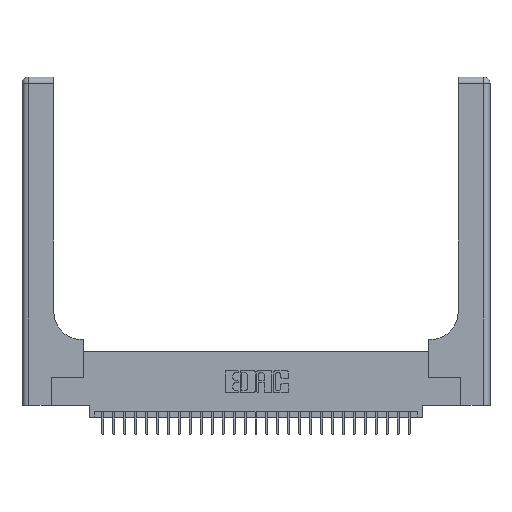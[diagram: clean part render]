
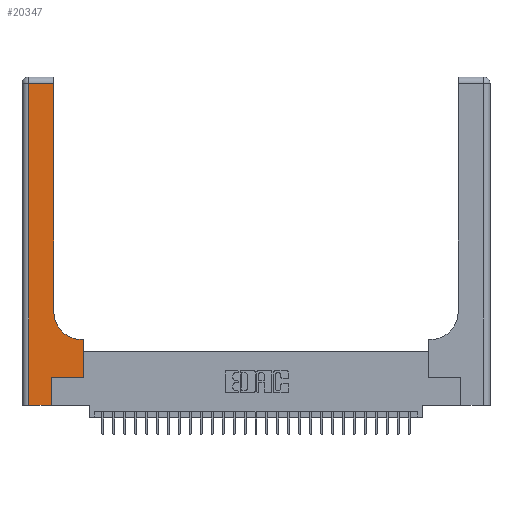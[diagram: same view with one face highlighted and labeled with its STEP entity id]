
A CAD part, top view. The second image highlights one B-rep face of the part: STEP entity #20347.
In plain terms, the highlighted planar face has unit normal (0, 0, 1).
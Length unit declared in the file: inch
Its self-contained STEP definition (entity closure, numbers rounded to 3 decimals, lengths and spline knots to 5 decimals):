
#326 = LINE ( 'NONE', #29440, #7261 ) ;
#518 = EDGE_CURVE ( 'NONE', #10290, #24856, #24675, .T. ) ;
#959 = LINE ( 'NONE', #28131, #12594 ) ;
#1615 = VECTOR ( 'NONE', #16192, 39.37008 ) ;
#1646 = VECTOR ( 'NONE', #24032, 39.37008 ) ;
#2129 = LINE ( 'NONE', #29507, #24504 ) ;
#3567 = PLANE ( 'NONE',  #21079 ) ;
#3671 = DIRECTION ( 'NONE',  ( 0., 0., -1. ) ) ;
#4589 = DIRECTION ( 'NONE',  ( 0., 1., 0. ) ) ;
#5098 = VERTEX_POINT ( 'NONE', #20747 ) ;
#5239 = AXIS2_PLACEMENT_3D ( 'NONE', #12744, #28800, #15045 ) ;
#5440 = VERTEX_POINT ( 'NONE', #18250 ) ;
#5540 = VERTEX_POINT ( 'NONE', #24027 ) ;
#5612 = CARTESIAN_POINT ( 'NONE',  ( 0.5585, 0.25, 0.37 ) ) ;
#5818 = FACE_OUTER_BOUND ( 'NONE', #27061, .T. ) ;
#6309 = VECTOR ( 'NONE', #28393, 39.37008 ) ;
#6556 = DIRECTION ( 'NONE',  ( -1., 0., 0. ) ) ;
#6905 = CARTESIAN_POINT ( 'NONE',  ( 0.269, 0.25, 0.37 ) ) ;
#7261 = VECTOR ( 'NONE', #15687, 39.37008 ) ;
#7595 = LINE ( 'NONE', #15906, #19853 ) ;
#7803 = LINE ( 'NONE', #6905, #1615 ) ;
#7983 = ORIENTED_EDGE ( 'NONE', *, *, #24202, .T. ) ;
#8025 = ORIENTED_EDGE ( 'NONE', *, *, #20539, .T. ) ;
#8749 = VERTEX_POINT ( 'NONE', #12777 ) ;
#9115 = ORIENTED_EDGE ( 'NONE', *, *, #15377, .T. ) ;
#9127 = ORIENTED_EDGE ( 'NONE', *, *, #18694, .T. ) ;
#9358 = EDGE_CURVE ( 'NONE', #5440, #18376, #28609, .T. ) ;
#10228 = ORIENTED_EDGE ( 'NONE', *, *, #9358, .T. ) ;
#10290 = VERTEX_POINT ( 'NONE', #22815 ) ;
#12074 = DIRECTION ( 'NONE',  ( 0., 1., 0. ) ) ;
#12594 = VECTOR ( 'NONE', #12074, 39.37008 ) ;
#12744 = CARTESIAN_POINT ( 'NONE',  ( 0.5415, 0.85, 0.37 ) ) ;
#12777 = CARTESIAN_POINT ( 'NONE',  ( 0.2915, 2.94, 0.37 ) ) ;
#13339 = CARTESIAN_POINT ( 'NONE',  ( 0.269, 0., 0.37 ) ) ;
#13676 = EDGE_CURVE ( 'NONE', #23272, #5098, #24753, .T. ) ;
#13821 = ORIENTED_EDGE ( 'NONE', *, *, #518, .T. ) ;
#13868 = LINE ( 'NONE', #18434, #26075 ) ;
#14112 = EDGE_CURVE ( 'NONE', #5540, #23272, #7803, .T. ) ;
#14633 = CARTESIAN_POINT ( 'NONE',  ( 0.5585, 0.25, 0.37 ) ) ;
#14650 = CARTESIAN_POINT ( 'NONE',  ( 0., 0., 0.37 ) ) ;
#15045 = DIRECTION ( 'NONE',  ( 1., 0., 0. ) ) ;
#15209 = CARTESIAN_POINT ( 'NONE',  ( 0., 3., 0.37 ) ) ;
#15377 = EDGE_CURVE ( 'NONE', #18376, #8749, #959, .T. ) ;
#15687 = DIRECTION ( 'NONE',  ( 0., -1., 0. ) ) ;
#15906 = CARTESIAN_POINT ( 'NONE',  ( 0., 2.94, 0.37 ) ) ;
#16192 = DIRECTION ( 'NONE',  ( 1., 0., 0. ) ) ;
#18250 = CARTESIAN_POINT ( 'NONE',  ( 0.5415, 0.6, 0.37 ) ) ;
#18376 = VERTEX_POINT ( 'NONE', #26567 ) ;
#18434 = CARTESIAN_POINT ( 'NONE',  ( 0.269, 0., 0.37 ) ) ;
#18694 = EDGE_CURVE ( 'NONE', #24856, #5540, #13868, .T. ) ;
#19668 = CARTESIAN_POINT ( 'NONE',  ( 0.06, 2.94, 0.37 ) ) ;
#19828 = DIRECTION ( 'NONE',  ( -1., 0., 0. ) ) ;
#19853 = VECTOR ( 'NONE', #29660, 39.37008 ) ;
#20347 = ADVANCED_FACE ( 'NONE', ( #5818 ), #3567, .F. ) ;
#20539 = EDGE_CURVE ( 'NONE', #8749, #21551, #7595, .T. ) ;
#20747 = CARTESIAN_POINT ( 'NONE',  ( 0.5585, 0.6, 0.37 ) ) ;
#21079 = AXIS2_PLACEMENT_3D ( 'NONE', #15209, #3671, #19828 ) ;
#21551 = VERTEX_POINT ( 'NONE', #19668 ) ;
#22815 = CARTESIAN_POINT ( 'NONE',  ( 0.06, 0., 0.37 ) ) ;
#23272 = VERTEX_POINT ( 'NONE', #14633 ) ;
#23516 = ORIENTED_EDGE ( 'NONE', *, *, #13676, .T. ) ;
#24027 = CARTESIAN_POINT ( 'NONE',  ( 0.269, 0.25, 0.37 ) ) ;
#24032 = DIRECTION ( 'NONE',  ( 0., 1., 0. ) ) ;
#24202 = EDGE_CURVE ( 'NONE', #21551, #10290, #326, .T. ) ;
#24504 = VECTOR ( 'NONE', #6556, 39.37008 ) ;
#24675 = LINE ( 'NONE', #14650, #6309 ) ;
#24753 = LINE ( 'NONE', #5612, #1646 ) ;
#24856 = VERTEX_POINT ( 'NONE', #13339 ) ;
#24899 = EDGE_CURVE ( 'NONE', #5098, #5440, #2129, .T. ) ;
#25684 = ORIENTED_EDGE ( 'NONE', *, *, #24899, .T. ) ;
#26075 = VECTOR ( 'NONE', #4589, 39.37008 ) ;
#26567 = CARTESIAN_POINT ( 'NONE',  ( 0.2915, 0.85, 0.37 ) ) ;
#27061 = EDGE_LOOP ( 'NONE', ( #9115, #8025, #7983, #13821, #9127, #28910, #23516, #25684, #10228 ) ) ;
#28131 = CARTESIAN_POINT ( 'NONE',  ( 0.2915, 3., 0.37 ) ) ;
#28393 = DIRECTION ( 'NONE',  ( 1., 0., 0. ) ) ;
#28609 = CIRCLE ( 'NONE', #5239, 0.25 ) ;
#28800 = DIRECTION ( 'NONE',  ( 0., 0., -1. ) ) ;
#28910 = ORIENTED_EDGE ( 'NONE', *, *, #14112, .T. ) ;
#29440 = CARTESIAN_POINT ( 'NONE',  ( 0.06, 3., 0.37 ) ) ;
#29507 = CARTESIAN_POINT ( 'NONE',  ( 0.2915, 0.6, 0.37 ) ) ;
#29660 = DIRECTION ( 'NONE',  ( -1., 0., 0. ) ) ;
